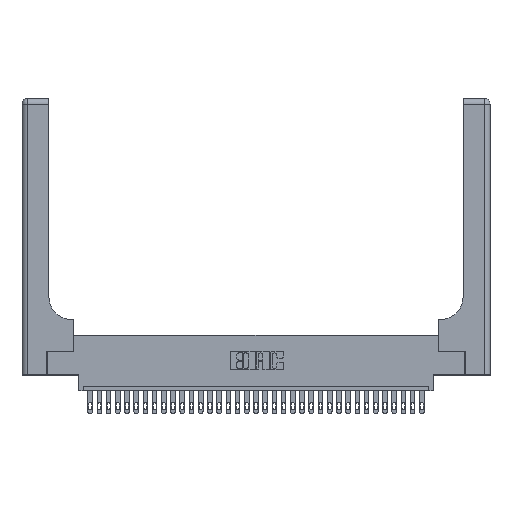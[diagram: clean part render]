
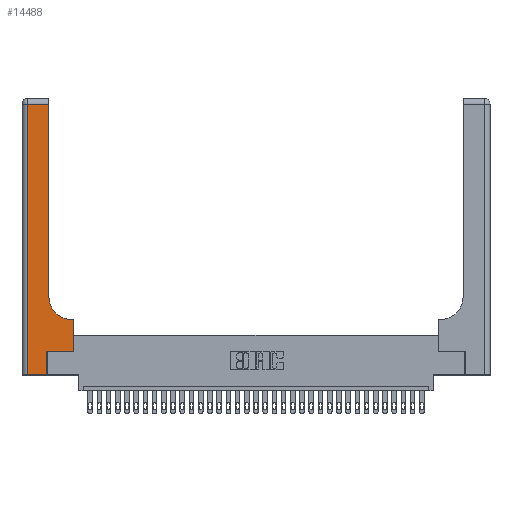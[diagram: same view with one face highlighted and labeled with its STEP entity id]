
A CAD part, top view. The second image highlights one B-rep face of the part: STEP entity #14488.
In plain terms, the highlighted planar face has unit normal (0, 0, 1).
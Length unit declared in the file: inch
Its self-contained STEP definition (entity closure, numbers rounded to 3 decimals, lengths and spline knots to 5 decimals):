
#82 = VECTOR ( 'NONE', #21145, 39.37008 ) ;
#494 = EDGE_LOOP ( 'NONE', ( #28838, #8316, #28900, #919, #12376, #28669, #6149, #15146, #14318 ) ) ;
#919 = ORIENTED_EDGE ( 'NONE', *, *, #31728, .T. ) ;
#923 = LINE ( 'NONE', #8354, #82 ) ;
#1863 = EDGE_CURVE ( 'NONE', #29082, #3529, #31631, .T. ) ;
#2189 = EDGE_CURVE ( 'NONE', #33105, #7206, #22723, .T. ) ;
#2246 = CARTESIAN_POINT ( 'NONE',  ( 0.06, 3., 0.37 ) ) ;
#3529 = VERTEX_POINT ( 'NONE', #8658 ) ;
#4339 = VERTEX_POINT ( 'NONE', #10520 ) ;
#4507 = CARTESIAN_POINT ( 'NONE',  ( 0., 3., 0.37 ) ) ;
#4637 = EDGE_CURVE ( 'NONE', #7206, #29082, #20827, .T. ) ;
#4740 = CARTESIAN_POINT ( 'NONE',  ( 0.269, 0.25, 0.37 ) ) ;
#5949 = VERTEX_POINT ( 'NONE', #30904 ) ;
#6079 = AXIS2_PLACEMENT_3D ( 'NONE', #16842, #14567, #27626 ) ;
#6149 = ORIENTED_EDGE ( 'NONE', *, *, #4637, .T. ) ;
#6800 = LINE ( 'NONE', #28049, #12899 ) ;
#7206 = VERTEX_POINT ( 'NONE', #29148 ) ;
#7307 = VERTEX_POINT ( 'NONE', #17304 ) ;
#7994 = VECTOR ( 'NONE', #9768, 39.37008 ) ;
#8316 = ORIENTED_EDGE ( 'NONE', *, *, #28434, .T. ) ;
#8354 = CARTESIAN_POINT ( 'NONE',  ( 0., 2.94, 0.37 ) ) ;
#8658 = CARTESIAN_POINT ( 'NONE',  ( 0.5415, 0.6, 0.37 ) ) ;
#9372 = VECTOR ( 'NONE', #16265, 39.37008 ) ;
#9674 = CARTESIAN_POINT ( 'NONE',  ( 0.5585, 0.6, 0.37 ) ) ;
#9768 = DIRECTION ( 'NONE',  ( -1., 0., 0. ) ) ;
#10520 = CARTESIAN_POINT ( 'NONE',  ( 0.269, 0., 0.37 ) ) ;
#10836 = VECTOR ( 'NONE', #14649, 39.37008 ) ;
#10945 = CARTESIAN_POINT ( 'NONE',  ( 0.2915, 3., 0.37 ) ) ;
#11158 = VERTEX_POINT ( 'NONE', #23222 ) ;
#11417 = VECTOR ( 'NONE', #19610, 39.37008 ) ;
#11826 = LINE ( 'NONE', #2246, #9372 ) ;
#12008 = CARTESIAN_POINT ( 'NONE',  ( 0., 0., 0.37 ) ) ;
#12376 = ORIENTED_EDGE ( 'NONE', *, *, #31881, .T. ) ;
#12447 = LINE ( 'NONE', #10945, #25516 ) ;
#12743 = CARTESIAN_POINT ( 'NONE',  ( 0.2915, 0.6, 0.37 ) ) ;
#12899 = VECTOR ( 'NONE', #30652, 39.37008 ) ;
#14318 = ORIENTED_EDGE ( 'NONE', *, *, #18336, .T. ) ;
#14488 = ADVANCED_FACE ( 'NONE', ( #16358 ), #14911, .F. ) ;
#14567 = DIRECTION ( 'NONE',  ( 0., 0., -1. ) ) ;
#14649 = DIRECTION ( 'NONE',  ( 1., 0., 0. ) ) ;
#14911 = PLANE ( 'NONE',  #23918 ) ;
#14950 = VECTOR ( 'NONE', #32811, 39.37008 ) ;
#15014 = DIRECTION ( 'NONE',  ( 0., 0., -1. ) ) ;
#15146 = ORIENTED_EDGE ( 'NONE', *, *, #1863, .T. ) ;
#16265 = DIRECTION ( 'NONE',  ( 0., -1., 0. ) ) ;
#16358 = FACE_OUTER_BOUND ( 'NONE', #494, .T. ) ;
#16842 = CARTESIAN_POINT ( 'NONE',  ( 0.5415, 0.85, 0.37 ) ) ;
#17304 = CARTESIAN_POINT ( 'NONE',  ( 0.2915, 0.85, 0.37 ) ) ;
#17562 = EDGE_CURVE ( 'NONE', #7307, #11158, #12447, .T. ) ;
#18336 = EDGE_CURVE ( 'NONE', #3529, #7307, #32365, .T. ) ;
#19610 = DIRECTION ( 'NONE',  ( 0., 1., 0. ) ) ;
#20148 = DIRECTION ( 'NONE',  ( -1., 0., 0. ) ) ;
#20733 = EDGE_CURVE ( 'NONE', #5949, #33068, #11826, .T. ) ;
#20827 = LINE ( 'NONE', #26425, #11417 ) ;
#21145 = DIRECTION ( 'NONE',  ( -1., 0., 0. ) ) ;
#22723 = LINE ( 'NONE', #32575, #14950 ) ;
#23222 = CARTESIAN_POINT ( 'NONE',  ( 0.2915, 2.94, 0.37 ) ) ;
#23918 = AXIS2_PLACEMENT_3D ( 'NONE', #4507, #15014, #20148 ) ;
#25154 = LINE ( 'NONE', #12008, #10836 ) ;
#25516 = VECTOR ( 'NONE', #29167, 39.37008 ) ;
#26425 = CARTESIAN_POINT ( 'NONE',  ( 0.5585, 0.25, 0.37 ) ) ;
#27626 = DIRECTION ( 'NONE',  ( 1., 0., 0. ) ) ;
#28049 = CARTESIAN_POINT ( 'NONE',  ( 0.269, 0., 0.37 ) ) ;
#28434 = EDGE_CURVE ( 'NONE', #11158, #5949, #923, .T. ) ;
#28669 = ORIENTED_EDGE ( 'NONE', *, *, #2189, .T. ) ;
#28838 = ORIENTED_EDGE ( 'NONE', *, *, #17562, .T. ) ;
#28900 = ORIENTED_EDGE ( 'NONE', *, *, #20733, .T. ) ;
#29082 = VERTEX_POINT ( 'NONE', #9674 ) ;
#29148 = CARTESIAN_POINT ( 'NONE',  ( 0.5585, 0.25, 0.37 ) ) ;
#29167 = DIRECTION ( 'NONE',  ( 0., 1., 0. ) ) ;
#30362 = CARTESIAN_POINT ( 'NONE',  ( 0.06, 0., 0.37 ) ) ;
#30652 = DIRECTION ( 'NONE',  ( 0., 1., 0. ) ) ;
#30904 = CARTESIAN_POINT ( 'NONE',  ( 0.06, 2.94, 0.37 ) ) ;
#31631 = LINE ( 'NONE', #12743, #7994 ) ;
#31728 = EDGE_CURVE ( 'NONE', #33068, #4339, #25154, .T. ) ;
#31881 = EDGE_CURVE ( 'NONE', #4339, #33105, #6800, .T. ) ;
#32365 = CIRCLE ( 'NONE', #6079, 0.25 ) ;
#32575 = CARTESIAN_POINT ( 'NONE',  ( 0.269, 0.25, 0.37 ) ) ;
#32811 = DIRECTION ( 'NONE',  ( 1., 0., 0. ) ) ;
#33068 = VERTEX_POINT ( 'NONE', #30362 ) ;
#33105 = VERTEX_POINT ( 'NONE', #4740 ) ;
